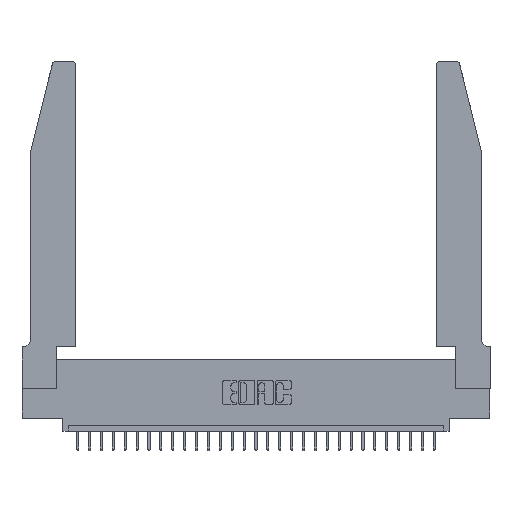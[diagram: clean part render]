
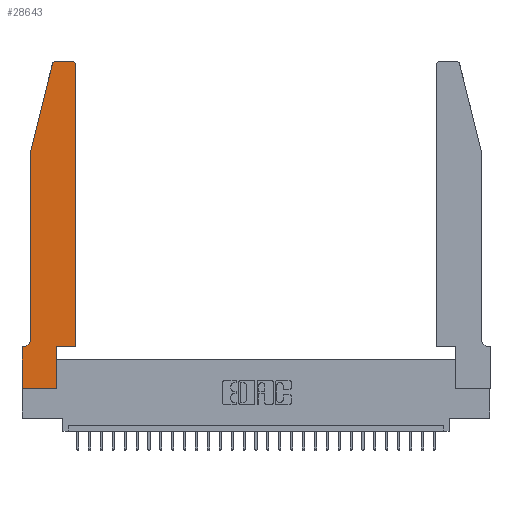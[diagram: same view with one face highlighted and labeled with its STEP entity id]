
A CAD part, top view. The second image highlights one B-rep face of the part: STEP entity #28643.
In plain terms, the highlighted planar face has unit normal (0, 0, 1).
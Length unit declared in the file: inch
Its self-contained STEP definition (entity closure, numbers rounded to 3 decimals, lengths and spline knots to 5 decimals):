
#433 = CARTESIAN_POINT ( 'NONE',  ( 0.0055, 0.35, 0.37 ) ) ;
#689 = ORIENTED_EDGE ( 'NONE', *, *, #11398, .T. ) ;
#746 = CARTESIAN_POINT ( 'NONE',  ( 0.0055, 0.42, 0.37 ) ) ;
#771 = VECTOR ( 'NONE', #2934, 39.37008 ) ;
#801 = AXIS2_PLACEMENT_3D ( 'NONE', #6429, #12972, #15366 ) ;
#828 = VECTOR ( 'NONE', #28822, 39.37008 ) ;
#946 = CARTESIAN_POINT ( 'NONE',  ( 0., 0.35, 0.37 ) ) ;
#952 = DIRECTION ( 'NONE',  ( 0., 1., 0. ) ) ;
#1090 = CARTESIAN_POINT ( 'NONE',  ( 0.25487, 2.72718, 0.37 ) ) ;
#1516 = CARTESIAN_POINT ( 'NONE',  ( 0.0755, 2., 0.37 ) ) ;
#1924 = DIRECTION ( 'NONE',  ( 0., 0., 1. ) ) ;
#2113 = CARTESIAN_POINT ( 'NONE',  ( 0.2605, 2.75, 0.37 ) ) ;
#2709 = EDGE_CURVE ( 'NONE', #8326, #17253, #4792, .T. ) ;
#2868 = CARTESIAN_POINT ( 'NONE',  ( 0.284, 2.72, 0.37 ) ) ;
#2926 = ORIENTED_EDGE ( 'NONE', *, *, #16567, .T. ) ;
#2934 = DIRECTION ( 'NONE',  ( 0., 1., 0. ) ) ;
#2949 = VERTEX_POINT ( 'NONE', #1090 ) ;
#3552 = DIRECTION ( 'NONE',  ( 1., 0., 0. ) ) ;
#3651 = CARTESIAN_POINT ( 'NONE',  ( 0., 0., 0.37 ) ) ;
#4327 = CIRCLE ( 'NONE', #28790, 0.03 ) ;
#4428 = CARTESIAN_POINT ( 'NONE',  ( 0., 0., 0.37 ) ) ;
#4792 = LINE ( 'NONE', #8280, #20652 ) ;
#5233 = CARTESIAN_POINT ( 'NONE',  ( 0.2865, 0.35, 0.37 ) ) ;
#5304 = VECTOR ( 'NONE', #10080, 39.37008 ) ;
#5402 = EDGE_CURVE ( 'NONE', #2949, #22090, #13383, .T. ) ;
#6128 = PLANE ( 'NONE',  #801 ) ;
#6176 = DIRECTION ( 'NONE',  ( 1., 0., 0. ) ) ;
#6280 = CARTESIAN_POINT ( 'NONE',  ( 0.4505, 0.35, 0.37 ) ) ;
#6429 = CARTESIAN_POINT ( 'NONE',  ( 0., 0.35, 0.37 ) ) ;
#7030 = ORIENTED_EDGE ( 'NONE', *, *, #2709, .T. ) ;
#7465 = DIRECTION ( 'NONE',  ( 0., 0., 1. ) ) ;
#7568 = CARTESIAN_POINT ( 'NONE',  ( 0.0755, 0.35, 0.37 ) ) ;
#7589 = VECTOR ( 'NONE', #15252, 39.37008 ) ;
#7716 = VERTEX_POINT ( 'NONE', #14963 ) ;
#8104 = CARTESIAN_POINT ( 'NONE',  ( 0.2865, 0., 0.37 ) ) ;
#8184 = DIRECTION ( 'NONE',  ( 0., -1., 0. ) ) ;
#8280 = CARTESIAN_POINT ( 'NONE',  ( 0., 0., 0.37 ) ) ;
#8326 = VERTEX_POINT ( 'NONE', #946 ) ;
#8773 = EDGE_CURVE ( 'NONE', #17535, #24973, #11532, .T. ) ;
#8882 = ORIENTED_EDGE ( 'NONE', *, *, #8773, .T. ) ;
#8928 = VERTEX_POINT ( 'NONE', #8104 ) ;
#9061 = LINE ( 'NONE', #5233, #771 ) ;
#9078 = ORIENTED_EDGE ( 'NONE', *, *, #28018, .T. ) ;
#9897 = DIRECTION ( 'NONE',  ( -1., 0., 0. ) ) ;
#9966 = CARTESIAN_POINT ( 'NONE',  ( 0.2865, 0.35, 0.37 ) ) ;
#10080 = DIRECTION ( 'NONE',  ( -1., 0., 0. ) ) ;
#10912 = EDGE_CURVE ( 'NONE', #18195, #8326, #17539, .T. ) ;
#11065 = ORIENTED_EDGE ( 'NONE', *, *, #19203, .T. ) ;
#11075 = CIRCLE ( 'NONE', #21144, 0.03 ) ;
#11398 = EDGE_CURVE ( 'NONE', #23471, #17535, #11075, .T. ) ;
#11532 = LINE ( 'NONE', #2113, #14367 ) ;
#11978 = VECTOR ( 'NONE', #6176, 39.37008 ) ;
#11994 = LINE ( 'NONE', #26092, #12334 ) ;
#12334 = VECTOR ( 'NONE', #952, 39.37008 ) ;
#12972 = DIRECTION ( 'NONE',  ( 0., 0., 1. ) ) ;
#13350 = CARTESIAN_POINT ( 'NONE',  ( 0.4205, 2.75, 0.37 ) ) ;
#13354 = CARTESIAN_POINT ( 'NONE',  ( 0.4505, 0.35, 0.37 ) ) ;
#13383 = LINE ( 'NONE', #1516, #7589 ) ;
#13703 = LINE ( 'NONE', #3651, #16540 ) ;
#14008 = DIRECTION ( 'NONE',  ( 1., 0., 0. ) ) ;
#14367 = VECTOR ( 'NONE', #18540, 39.37008 ) ;
#14636 = EDGE_CURVE ( 'NONE', #29565, #25072, #25309, .T. ) ;
#14745 = ORIENTED_EDGE ( 'NONE', *, *, #25965, .T. ) ;
#14963 = CARTESIAN_POINT ( 'NONE',  ( 0.0755, 0.42, 0.37 ) ) ;
#15252 = DIRECTION ( 'NONE',  ( -0.239, -0.971, 0. ) ) ;
#15366 = DIRECTION ( 'NONE',  ( 1., 0., 0. ) ) ;
#15761 = EDGE_CURVE ( 'NONE', #8928, #29565, #9061, .T. ) ;
#16540 = VECTOR ( 'NONE', #3552, 39.37008 ) ;
#16567 = EDGE_CURVE ( 'NONE', #24973, #2949, #4327, .T. ) ;
#17253 = VERTEX_POINT ( 'NONE', #4428 ) ;
#17535 = VERTEX_POINT ( 'NONE', #13350 ) ;
#17539 = LINE ( 'NONE', #7568, #5304 ) ;
#17755 = CARTESIAN_POINT ( 'NONE',  ( 0.0755, 2., 0.37 ) ) ;
#18058 = DIRECTION ( 'NONE',  ( 1., 0., 0. ) ) ;
#18195 = VERTEX_POINT ( 'NONE', #433 ) ;
#18540 = DIRECTION ( 'NONE',  ( -1., 0., 0. ) ) ;
#19190 = AXIS2_PLACEMENT_3D ( 'NONE', #746, #23881, #9897 ) ;
#19203 = EDGE_CURVE ( 'NONE', #7716, #18195, #25843, .T. ) ;
#20652 = VECTOR ( 'NONE', #8184, 39.37008 ) ;
#21144 = AXIS2_PLACEMENT_3D ( 'NONE', #21899, #1924, #18058 ) ;
#21899 = CARTESIAN_POINT ( 'NONE',  ( 0.4205, 2.72, 0.37 ) ) ;
#21986 = CARTESIAN_POINT ( 'NONE',  ( 0.0755, 2., 0.37 ) ) ;
#22090 = VERTEX_POINT ( 'NONE', #17755 ) ;
#22391 = CARTESIAN_POINT ( 'NONE',  ( 0.284, 2.75, 0.37 ) ) ;
#22586 = EDGE_CURVE ( 'NONE', #22090, #7716, #29211, .T. ) ;
#23173 = ORIENTED_EDGE ( 'NONE', *, *, #5402, .T. ) ;
#23471 = VERTEX_POINT ( 'NONE', #23567 ) ;
#23567 = CARTESIAN_POINT ( 'NONE',  ( 0.4505, 2.72, 0.37 ) ) ;
#23709 = FACE_OUTER_BOUND ( 'NONE', #26752, .T. ) ;
#23881 = DIRECTION ( 'NONE',  ( 0., 0., -1. ) ) ;
#24774 = ORIENTED_EDGE ( 'NONE', *, *, #14636, .T. ) ;
#24973 = VERTEX_POINT ( 'NONE', #22391 ) ;
#25072 = VERTEX_POINT ( 'NONE', #13354 ) ;
#25309 = LINE ( 'NONE', #6280, #11978 ) ;
#25843 = CIRCLE ( 'NONE', #19190, 0.07 ) ;
#25965 = EDGE_CURVE ( 'NONE', #25072, #23471, #11994, .T. ) ;
#26033 = ORIENTED_EDGE ( 'NONE', *, *, #15761, .T. ) ;
#26092 = CARTESIAN_POINT ( 'NONE',  ( 0.4505, 0.35, 0.37 ) ) ;
#26455 = ORIENTED_EDGE ( 'NONE', *, *, #22586, .T. ) ;
#26752 = EDGE_LOOP ( 'NONE', ( #8882, #2926, #23173, #26455, #11065, #29249, #7030, #9078, #26033, #24774, #14745, #689 ) ) ;
#28018 = EDGE_CURVE ( 'NONE', #17253, #8928, #13703, .T. ) ;
#28643 = ADVANCED_FACE ( 'NONE', ( #23709 ), #6128, .T. ) ;
#28790 = AXIS2_PLACEMENT_3D ( 'NONE', #2868, #7465, #14008 ) ;
#28822 = DIRECTION ( 'NONE',  ( 0., -1., 0. ) ) ;
#29211 = LINE ( 'NONE', #21986, #828 ) ;
#29249 = ORIENTED_EDGE ( 'NONE', *, *, #10912, .T. ) ;
#29565 = VERTEX_POINT ( 'NONE', #9966 ) ;
